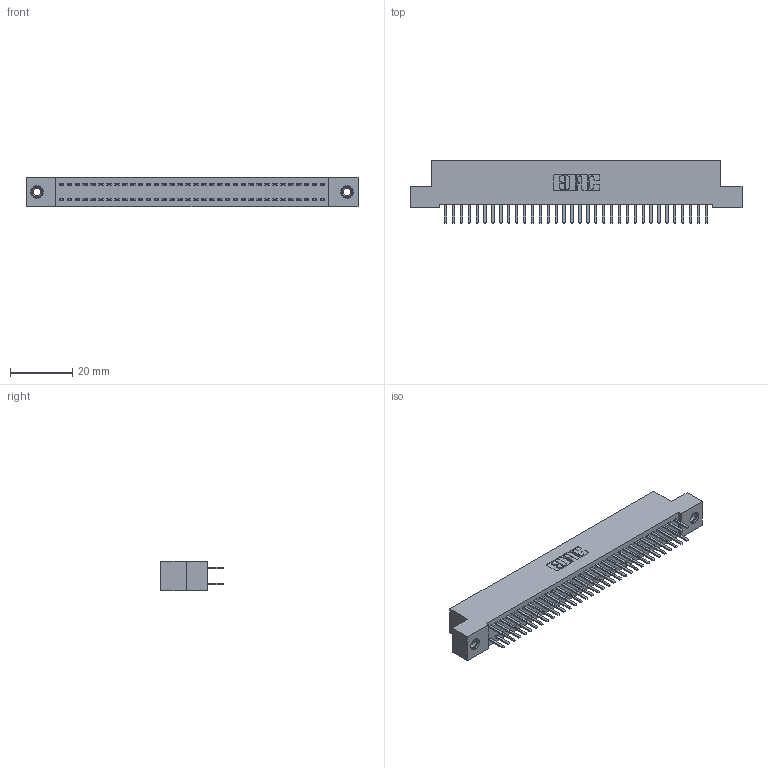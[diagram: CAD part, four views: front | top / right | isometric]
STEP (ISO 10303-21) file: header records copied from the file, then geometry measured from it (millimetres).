
FILE_DESCRIPTION (( 'STEP AP203' ), '1' );
FILE_NAME ('392-068-520-207.STEP', '2019-10-09T11:29:52', ( '' ), ( '' ), 'SwSTEP 2.0', 'SolidWorks 2016', '' );
FILE_SCHEMA (( 'CONFIG_CONTROL_DESIGN' ));
Length unit declared in the file: inch
Products named in the file (4): 345-250-001_345-250-005-103; 392-068-520-207; 342 Part_TI; 345-292-001_345-293-120
Assembly tree (71 placements, depth 2):
  392-068-520-207
    342 Part_TI
    345-292-001_345-293-120  x68
    345-250-001_345-250-005-103  x2
Bounding box: 106.68 x 20.02 x 9.4 mm (x, y, z)
Volume: 9504.7 mm3; surface area: 15229.5 mm2
Topology: 71 solids, 71 shells, 3978 faces, 11519 edges, 7490 vertices
Faces by surface type: plane 2682, cylinder 1280, cone 12, torus 4
Entity records: 24076 total; most frequent: CARTESIAN_POINT 3993, ORIENTED_EDGE 3910, DIRECTION 3445, EDGE_CURVE 1955, VECTOR 1803, LINE 1803, VERTEX_POINT 1296, AXIS2_PLACEMENT_3D 821
